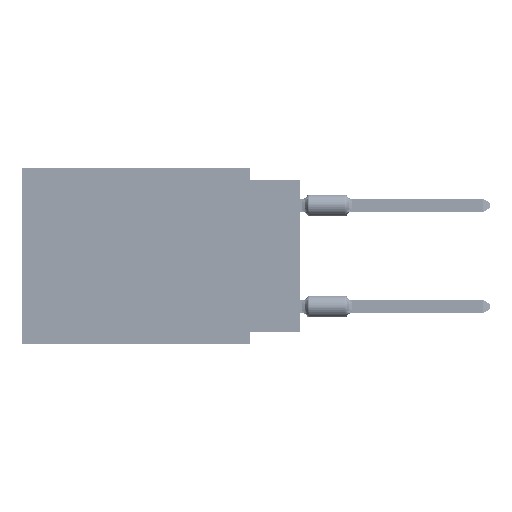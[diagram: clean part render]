
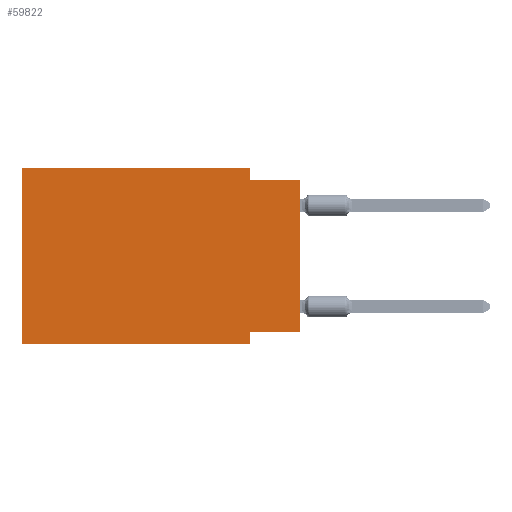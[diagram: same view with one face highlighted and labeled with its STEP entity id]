
A CAD part, left-side view. The second image highlights one B-rep face of the part: STEP entity #59822.
In plain terms, the highlighted planar face has unit normal (-1, 0, 0).
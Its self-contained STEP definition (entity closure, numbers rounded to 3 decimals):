
#532 = DIRECTION ( 'NONE',  ( 0., 0., -1. ) ) ;
#2371 = ORIENTED_EDGE ( 'NONE', *, *, #60484, .F. ) ;
#2611 = VECTOR ( 'NONE', #6701, 1000. ) ;
#3824 = AXIS2_PLACEMENT_3D ( 'NONE', #38907, #68876, #532 ) ;
#4271 = LINE ( 'NONE', #23264, #17991 ) ;
#4369 = CARTESIAN_POINT ( 'NONE',  ( 0., 0., -0.635 ) ) ;
#6701 = DIRECTION ( 'NONE',  ( 0., -1., 0. ) ) ;
#7728 = ORIENTED_EDGE ( 'NONE', *, *, #54693, .F. ) ;
#8137 = ORIENTED_EDGE ( 'NONE', *, *, #11783, .F. ) ;
#10362 = LINE ( 'NONE', #35822, #66717 ) ;
#10724 = CARTESIAN_POINT ( 'NONE',  ( 0., 2.54, -8.89 ) ) ;
#11007 = CARTESIAN_POINT ( 'NONE',  ( 0., 13.97, -8.89 ) ) ;
#11119 = CARTESIAN_POINT ( 'NONE',  ( 0., 13.97, -8.89 ) ) ;
#11660 = VECTOR ( 'NONE', #23710, 1000. ) ;
#11783 = EDGE_CURVE ( 'NONE', #45407, #27502, #53604, .T. ) ;
#12563 = ORIENTED_EDGE ( 'NONE', *, *, #50872, .F. ) ;
#12748 = CARTESIAN_POINT ( 'NONE',  ( 0., 13.97, 0. ) ) ;
#17991 = VECTOR ( 'NONE', #53212, 1000. ) ;
#19106 = FACE_OUTER_BOUND ( 'NONE', #51113, .T. ) ;
#20438 = VERTEX_POINT ( 'NONE', #4369 ) ;
#20932 = VERTEX_POINT ( 'NONE', #11119 ) ;
#21051 = ORIENTED_EDGE ( 'NONE', *, *, #69129, .F. ) ;
#22332 = EDGE_CURVE ( 'NONE', #65875, #20438, #63834, .T. ) ;
#23264 = CARTESIAN_POINT ( 'NONE',  ( 0., 2.54, 0. ) ) ;
#23710 = DIRECTION ( 'NONE',  ( 0., 0., 1. ) ) ;
#24450 = ORIENTED_EDGE ( 'NONE', *, *, #56953, .T. ) ;
#25152 = VERTEX_POINT ( 'NONE', #50921 ) ;
#26767 = VECTOR ( 'NONE', #48051, 1000. ) ;
#27322 = VECTOR ( 'NONE', #32697, 1000. ) ;
#27502 = VERTEX_POINT ( 'NONE', #33526 ) ;
#28404 = ORIENTED_EDGE ( 'NONE', *, *, #77110, .T. ) ;
#32697 = DIRECTION ( 'NONE',  ( 0., -1., 0. ) ) ;
#33526 = CARTESIAN_POINT ( 'NONE',  ( 0., 2.54, -8.89 ) ) ;
#33630 = CARTESIAN_POINT ( 'NONE',  ( 0., 13.97, 0. ) ) ;
#35822 = CARTESIAN_POINT ( 'NONE',  ( 0., 0., -8.255 ) ) ;
#36157 = CARTESIAN_POINT ( 'NONE',  ( 0., 2.54, 0. ) ) ;
#36408 = VERTEX_POINT ( 'NONE', #36157 ) ;
#38907 = CARTESIAN_POINT ( 'NONE',  ( 0., 13.97, 0. ) ) ;
#44290 = LINE ( 'NONE', #12748, #2611 ) ;
#45407 = VERTEX_POINT ( 'NONE', #67574 ) ;
#48051 = DIRECTION ( 'NONE',  ( 0., 0., 1. ) ) ;
#50872 = EDGE_CURVE ( 'NONE', #75400, #36408, #44290, .T. ) ;
#50921 = CARTESIAN_POINT ( 'NONE',  ( 0., 0., -8.255 ) ) ;
#51113 = EDGE_LOOP ( 'NONE', ( #24450, #60947, #21051, #12563, #2371, #28404, #8137, #7728 ) ) ;
#53212 = DIRECTION ( 'NONE',  ( 0., 0., -1. ) ) ;
#53604 = LINE ( 'NONE', #10724, #54520 ) ;
#54213 = CARTESIAN_POINT ( 'NONE',  ( 0., 2.54, -0.635 ) ) ;
#54289 = DIRECTION ( 'NONE',  ( 0., -1., 0. ) ) ;
#54520 = VECTOR ( 'NONE', #78685, 1000. ) ;
#54693 = EDGE_CURVE ( 'NONE', #25152, #45407, #10362, .T. ) ;
#54826 = DIRECTION ( 'NONE',  ( 0., 1., 0. ) ) ;
#56953 = EDGE_CURVE ( 'NONE', #25152, #20438, #71931, .T. ) ;
#58959 = CARTESIAN_POINT ( 'NONE',  ( 0., 0., -0.635 ) ) ;
#59822 = ADVANCED_FACE ( 'NONE', ( #19106 ), #75740, .F. ) ;
#60484 = EDGE_CURVE ( 'NONE', #20932, #75400, #73461, .T. ) ;
#60947 = ORIENTED_EDGE ( 'NONE', *, *, #22332, .F. ) ;
#60975 = CARTESIAN_POINT ( 'NONE',  ( 0., 0., 0. ) ) ;
#61152 = LINE ( 'NONE', #11007, #69211 ) ;
#63834 = LINE ( 'NONE', #58959, #27322 ) ;
#65875 = VERTEX_POINT ( 'NONE', #54213 ) ;
#66717 = VECTOR ( 'NONE', #54826, 1000. ) ;
#67380 = CARTESIAN_POINT ( 'NONE',  ( 0., 13.97, 0. ) ) ;
#67574 = CARTESIAN_POINT ( 'NONE',  ( 0., 2.54, -8.255 ) ) ;
#68876 = DIRECTION ( 'NONE',  ( 1., 0., 0. ) ) ;
#69129 = EDGE_CURVE ( 'NONE', #36408, #65875, #4271, .T. ) ;
#69211 = VECTOR ( 'NONE', #54289, 1000. ) ;
#71931 = LINE ( 'NONE', #60975, #26767 ) ;
#73461 = LINE ( 'NONE', #67380, #11660 ) ;
#75400 = VERTEX_POINT ( 'NONE', #33630 ) ;
#75740 = PLANE ( 'NONE',  #3824 ) ;
#77110 = EDGE_CURVE ( 'NONE', #20932, #27502, #61152, .T. ) ;
#78685 = DIRECTION ( 'NONE',  ( 0., 0., -1. ) ) ;
